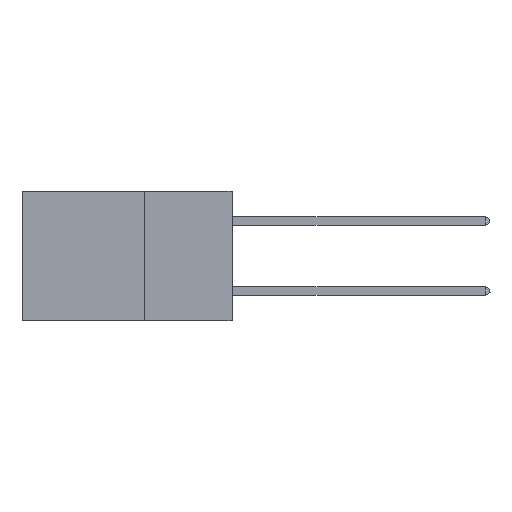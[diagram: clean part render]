
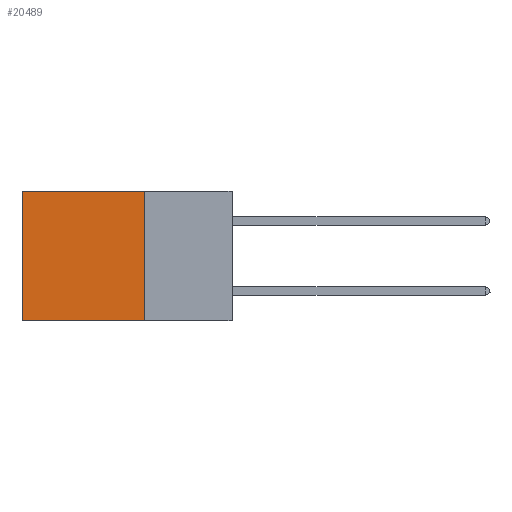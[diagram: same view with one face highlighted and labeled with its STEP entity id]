
A CAD part, left-side view. The second image highlights one B-rep face of the part: STEP entity #20489.
In plain terms, the highlighted planar face has unit normal (-1, 0, 0).
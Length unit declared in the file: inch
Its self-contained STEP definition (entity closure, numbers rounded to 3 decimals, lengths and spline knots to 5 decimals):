
#3063 = DIRECTION ( 'NONE',  ( 0., 1., 0. ) ) ;
#4486 = CARTESIAN_POINT ( 'NONE',  ( 0.2875, 0.6, 0. ) ) ;
#6396 = DIRECTION ( 'NONE',  ( 0., 0., -1. ) ) ;
#7341 = VERTEX_POINT ( 'NONE', #4486 ) ;
#8342 = LINE ( 'NONE', #33527, #40681 ) ;
#9955 = PLANE ( 'NONE',  #41350 ) ;
#10188 = DIRECTION ( 'NONE',  ( 0., 1., 0. ) ) ;
#11294 = EDGE_CURVE ( 'NONE', #35727, #13478, #17228, .T. ) ;
#11440 = CARTESIAN_POINT ( 'NONE',  ( 0.2875, 0.6, -0.37 ) ) ;
#11851 = EDGE_CURVE ( 'NONE', #35727, #7341, #37732, .T. ) ;
#12021 = VECTOR ( 'NONE', #3063, 39.37008 ) ;
#13045 = ORIENTED_EDGE ( 'NONE', *, *, #27114, .T. ) ;
#13285 = DIRECTION ( 'NONE',  ( 0., 0., -1. ) ) ;
#13478 = VERTEX_POINT ( 'NONE', #34199 ) ;
#13840 = ORIENTED_EDGE ( 'NONE', *, *, #11294, .F. ) ;
#16201 = VECTOR ( 'NONE', #6396, 39.37008 ) ;
#17228 = LINE ( 'NONE', #29112, #16201 ) ;
#18079 = VERTEX_POINT ( 'NONE', #11440 ) ;
#19421 = CARTESIAN_POINT ( 'NONE',  ( 0.2875, 0.25, 0. ) ) ;
#19695 = DIRECTION ( 'NONE',  ( 1., 0., 0. ) ) ;
#20004 = VECTOR ( 'NONE', #10188, 39.37008 ) ;
#20489 = ADVANCED_FACE ( 'NONE', ( #40613 ), #9955, .F. ) ;
#20862 = CARTESIAN_POINT ( 'NONE',  ( 0.2875, 0.25, 0. ) ) ;
#21224 = EDGE_CURVE ( 'NONE', #13478, #18079, #28511, .T. ) ;
#26126 = CARTESIAN_POINT ( 'NONE',  ( 0.2875, 0.25, 0. ) ) ;
#26301 = EDGE_LOOP ( 'NONE', ( #13045, #37854, #13840, #30332 ) ) ;
#27114 = EDGE_CURVE ( 'NONE', #7341, #18079, #8342, .T. ) ;
#28511 = LINE ( 'NONE', #39101, #20004 ) ;
#29112 = CARTESIAN_POINT ( 'NONE',  ( 0.2875, 0.25, 0. ) ) ;
#30332 = ORIENTED_EDGE ( 'NONE', *, *, #11851, .T. ) ;
#33527 = CARTESIAN_POINT ( 'NONE',  ( 0.2875, 0.6, 0. ) ) ;
#34199 = CARTESIAN_POINT ( 'NONE',  ( 0.2875, 0.25, -0.37 ) ) ;
#35727 = VERTEX_POINT ( 'NONE', #20862 ) ;
#37732 = LINE ( 'NONE', #19421, #12021 ) ;
#37854 = ORIENTED_EDGE ( 'NONE', *, *, #21224, .F. ) ;
#39101 = CARTESIAN_POINT ( 'NONE',  ( 0.2875, 0.25, -0.37 ) ) ;
#39967 = DIRECTION ( 'NONE',  ( 0., 0., -1. ) ) ;
#40613 = FACE_OUTER_BOUND ( 'NONE', #26301, .T. ) ;
#40681 = VECTOR ( 'NONE', #39967, 39.37008 ) ;
#41350 = AXIS2_PLACEMENT_3D ( 'NONE', #26126, #19695, #13285 ) ;
